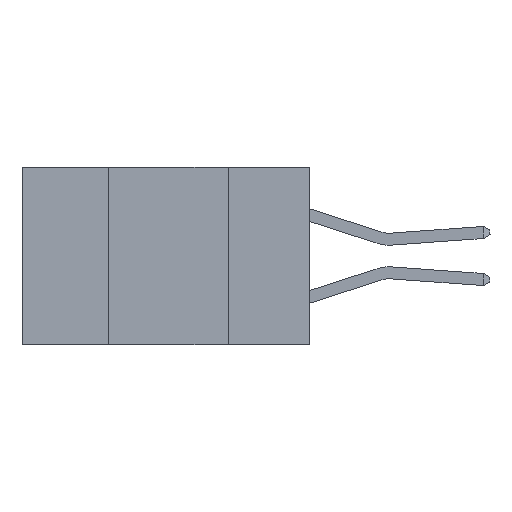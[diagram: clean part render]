
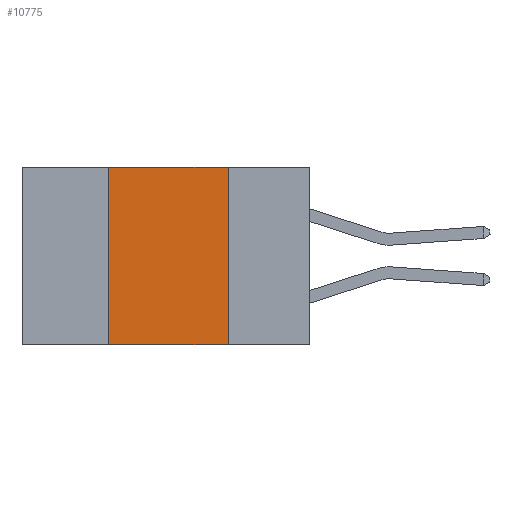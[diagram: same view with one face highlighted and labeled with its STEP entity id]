
A CAD part, left-side view. The second image highlights one B-rep face of the part: STEP entity #10775.
In plain terms, the highlighted planar face has unit normal (-1, 0, 0).
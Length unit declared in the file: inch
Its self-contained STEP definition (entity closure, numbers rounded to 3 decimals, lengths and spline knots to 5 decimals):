
#91 = AXIS2_PLACEMENT_3D ( 'NONE', #8686, #18714, #24970 ) ;
#824 = VECTOR ( 'NONE', #13558, 39.37008 ) ;
#2646 = CARTESIAN_POINT ( 'NONE',  ( 0., 0.17, -0.37 ) ) ;
#2861 = VECTOR ( 'NONE', #2971, 39.37008 ) ;
#2971 = DIRECTION ( 'NONE',  ( 0., -1., 0. ) ) ;
#3322 = LINE ( 'NONE', #4780, #3638 ) ;
#3600 = LINE ( 'NONE', #5677, #824 ) ;
#3638 = VECTOR ( 'NONE', #11233, 39.37008 ) ;
#3725 = VECTOR ( 'NONE', #6055, 39.37008 ) ;
#4780 = CARTESIAN_POINT ( 'NONE',  ( 0., 0.42, -0.37 ) ) ;
#5341 = VERTEX_POINT ( 'NONE', #19392 ) ;
#5677 = CARTESIAN_POINT ( 'NONE',  ( 0., 0.17, -0.37 ) ) ;
#5730 = EDGE_CURVE ( 'NONE', #5341, #24859, #12825, .T. ) ;
#6046 = VERTEX_POINT ( 'NONE', #10104 ) ;
#6055 = DIRECTION ( 'NONE',  ( 0., -1., 0. ) ) ;
#6374 = EDGE_CURVE ( 'NONE', #6046, #24859, #3600, .T. ) ;
#6433 = EDGE_CURVE ( 'NONE', #19534, #6046, #18140, .T. ) ;
#6809 = ORIENTED_EDGE ( 'NONE', *, *, #6374, .F. ) ;
#7816 = ORIENTED_EDGE ( 'NONE', *, *, #15257, .F. ) ;
#8427 = FACE_OUTER_BOUND ( 'NONE', #8832, .T. ) ;
#8686 = CARTESIAN_POINT ( 'NONE',  ( 0., 0.6, 0. ) ) ;
#8832 = EDGE_LOOP ( 'NONE', ( #6809, #20866, #7816, #16242 ) ) ;
#10104 = CARTESIAN_POINT ( 'NONE',  ( 0., 0.17, 0. ) ) ;
#10775 = ADVANCED_FACE ( 'NONE', ( #8427 ), #16353, .F. ) ;
#11233 = DIRECTION ( 'NONE',  ( 0., 0., 1. ) ) ;
#12825 = LINE ( 'NONE', #20808, #2861 ) ;
#13558 = DIRECTION ( 'NONE',  ( 0., 0., -1. ) ) ;
#14062 = CARTESIAN_POINT ( 'NONE',  ( 0., 0.6, 0. ) ) ;
#15257 = EDGE_CURVE ( 'NONE', #5341, #19534, #3322, .T. ) ;
#16242 = ORIENTED_EDGE ( 'NONE', *, *, #5730, .T. ) ;
#16353 = PLANE ( 'NONE',  #91 ) ;
#17226 = CARTESIAN_POINT ( 'NONE',  ( 0., 0.42, 0. ) ) ;
#18140 = LINE ( 'NONE', #14062, #3725 ) ;
#18714 = DIRECTION ( 'NONE',  ( 1., 0., 0. ) ) ;
#19392 = CARTESIAN_POINT ( 'NONE',  ( 0., 0.42, -0.37 ) ) ;
#19534 = VERTEX_POINT ( 'NONE', #17226 ) ;
#20808 = CARTESIAN_POINT ( 'NONE',  ( 0., 0.6, -0.37 ) ) ;
#20866 = ORIENTED_EDGE ( 'NONE', *, *, #6433, .F. ) ;
#24859 = VERTEX_POINT ( 'NONE', #2646 ) ;
#24970 = DIRECTION ( 'NONE',  ( 0., 0., -1. ) ) ;
